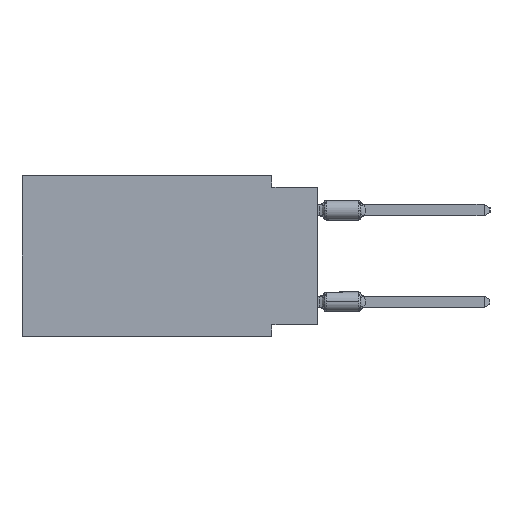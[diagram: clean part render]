
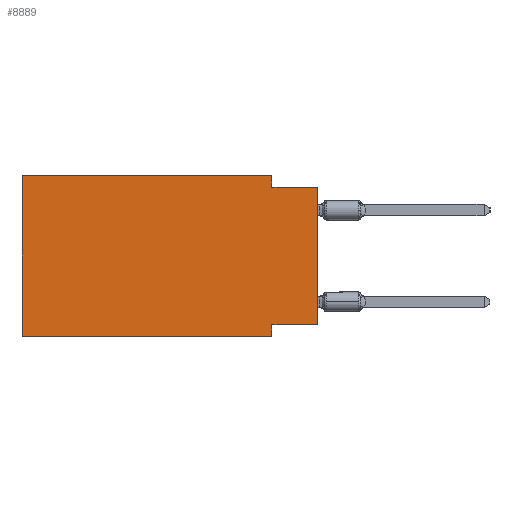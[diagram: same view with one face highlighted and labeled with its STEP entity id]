
A CAD part, left-side view. The second image highlights one B-rep face of the part: STEP entity #8889.
In plain terms, the highlighted planar face has unit normal (-1, 0, 0).
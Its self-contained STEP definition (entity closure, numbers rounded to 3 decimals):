
#313 = LINE ( 'NONE', #31589, #7486 ) ;
#1511 = VERTEX_POINT ( 'NONE', #18893 ) ;
#1699 = DIRECTION ( 'NONE',  ( 0., 0., -1. ) ) ;
#2192 = PLANE ( 'NONE',  #33524 ) ;
#2637 = CARTESIAN_POINT ( 'NONE',  ( 0., 0., -0.635 ) ) ;
#2842 = DIRECTION ( 'NONE',  ( 0., 0., 1. ) ) ;
#3196 = LINE ( 'NONE', #24272, #4653 ) ;
#3519 = EDGE_LOOP ( 'NONE', ( #17296, #11450, #19695, #19029, #26177, #29311, #13416, #9397 ) ) ;
#4653 = VECTOR ( 'NONE', #11479, 1000. ) ;
#4673 = CARTESIAN_POINT ( 'NONE',  ( 0., 2.54, -0.635 ) ) ;
#4777 = DIRECTION ( 'NONE',  ( 0., 0., -1. ) ) ;
#5159 = CARTESIAN_POINT ( 'NONE',  ( 0., 0., -8.255 ) ) ;
#5335 = DIRECTION ( 'NONE',  ( 0., -1., 0. ) ) ;
#5899 = VERTEX_POINT ( 'NONE', #6217 ) ;
#5930 = CARTESIAN_POINT ( 'NONE',  ( 0., 2.54, -8.89 ) ) ;
#6217 = CARTESIAN_POINT ( 'NONE',  ( 0., 16.383, -8.89 ) ) ;
#6484 = VECTOR ( 'NONE', #2842, 1000. ) ;
#7486 = VECTOR ( 'NONE', #5335, 1000. ) ;
#7544 = DIRECTION ( 'NONE',  ( 1., 0., 0. ) ) ;
#8195 = VECTOR ( 'NONE', #9191, 1000. ) ;
#8300 = CARTESIAN_POINT ( 'NONE',  ( 0., 0., -0.635 ) ) ;
#8691 = LINE ( 'NONE', #5930, #17707 ) ;
#8889 = ADVANCED_FACE ( 'NONE', ( #10130 ), #2192, .F. ) ;
#9191 = DIRECTION ( 'NONE',  ( 0., 1., 0. ) ) ;
#9397 = ORIENTED_EDGE ( 'NONE', *, *, #10370, .F. ) ;
#10130 = FACE_OUTER_BOUND ( 'NONE', #3519, .T. ) ;
#10370 = EDGE_CURVE ( 'NONE', #27900, #29808, #19234, .T. ) ;
#11450 = ORIENTED_EDGE ( 'NONE', *, *, #25141, .F. ) ;
#11479 = DIRECTION ( 'NONE',  ( 0., -1., 0. ) ) ;
#11626 = EDGE_CURVE ( 'NONE', #29808, #1511, #8691, .T. ) ;
#12919 = CARTESIAN_POINT ( 'NONE',  ( 0., 16.383, 0. ) ) ;
#13300 = LINE ( 'NONE', #8300, #21170 ) ;
#13416 = ORIENTED_EDGE ( 'NONE', *, *, #11626, .F. ) ;
#15981 = CARTESIAN_POINT ( 'NONE',  ( 0., 0., 0. ) ) ;
#17208 = CARTESIAN_POINT ( 'NONE',  ( 0., 2.54, -8.255 ) ) ;
#17296 = ORIENTED_EDGE ( 'NONE', *, *, #19024, .T. ) ;
#17424 = CARTESIAN_POINT ( 'NONE',  ( 0., 2.54, 0. ) ) ;
#17656 = DIRECTION ( 'NONE',  ( 0., 0., 1. ) ) ;
#17707 = VECTOR ( 'NONE', #19239, 1000. ) ;
#18893 = CARTESIAN_POINT ( 'NONE',  ( 0., 2.54, -8.89 ) ) ;
#18951 = VECTOR ( 'NONE', #1699, 1000. ) ;
#19024 = EDGE_CURVE ( 'NONE', #27900, #26288, #31691, .T. ) ;
#19029 = ORIENTED_EDGE ( 'NONE', *, *, #29256, .F. ) ;
#19234 = LINE ( 'NONE', #24565, #8195 ) ;
#19239 = DIRECTION ( 'NONE',  ( 0., 0., -1. ) ) ;
#19582 = VERTEX_POINT ( 'NONE', #12919 ) ;
#19695 = ORIENTED_EDGE ( 'NONE', *, *, #25417, .F. ) ;
#20521 = LINE ( 'NONE', #17424, #18951 ) ;
#21170 = VECTOR ( 'NONE', #23832, 1000. ) ;
#21592 = VERTEX_POINT ( 'NONE', #22552 ) ;
#22552 = CARTESIAN_POINT ( 'NONE',  ( 0., 2.54, 0. ) ) ;
#22823 = LINE ( 'NONE', #27516, #32341 ) ;
#23832 = DIRECTION ( 'NONE',  ( 0., -1., 0. ) ) ;
#24272 = CARTESIAN_POINT ( 'NONE',  ( 0., 16.383, -8.89 ) ) ;
#24565 = CARTESIAN_POINT ( 'NONE',  ( 0., 0., -8.255 ) ) ;
#25141 = EDGE_CURVE ( 'NONE', #32813, #26288, #13300, .T. ) ;
#25417 = EDGE_CURVE ( 'NONE', #21592, #32813, #20521, .T. ) ;
#26032 = EDGE_CURVE ( 'NONE', #5899, #1511, #3196, .T. ) ;
#26177 = ORIENTED_EDGE ( 'NONE', *, *, #33768, .F. ) ;
#26288 = VERTEX_POINT ( 'NONE', #2637 ) ;
#27516 = CARTESIAN_POINT ( 'NONE',  ( 0., 16.383, 0. ) ) ;
#27900 = VERTEX_POINT ( 'NONE', #5159 ) ;
#29256 = EDGE_CURVE ( 'NONE', #19582, #21592, #313, .T. ) ;
#29311 = ORIENTED_EDGE ( 'NONE', *, *, #26032, .T. ) ;
#29808 = VERTEX_POINT ( 'NONE', #17208 ) ;
#31589 = CARTESIAN_POINT ( 'NONE',  ( 0., 16.383, 0. ) ) ;
#31691 = LINE ( 'NONE', #15981, #6484 ) ;
#32341 = VECTOR ( 'NONE', #17656, 1000. ) ;
#32813 = VERTEX_POINT ( 'NONE', #4673 ) ;
#33287 = CARTESIAN_POINT ( 'NONE',  ( 0., 16.383, 0. ) ) ;
#33524 = AXIS2_PLACEMENT_3D ( 'NONE', #33287, #7544, #4777 ) ;
#33768 = EDGE_CURVE ( 'NONE', #5899, #19582, #22823, .T. ) ;
